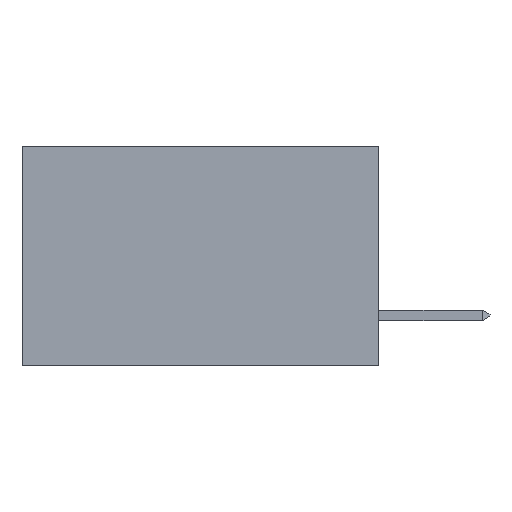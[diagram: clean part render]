
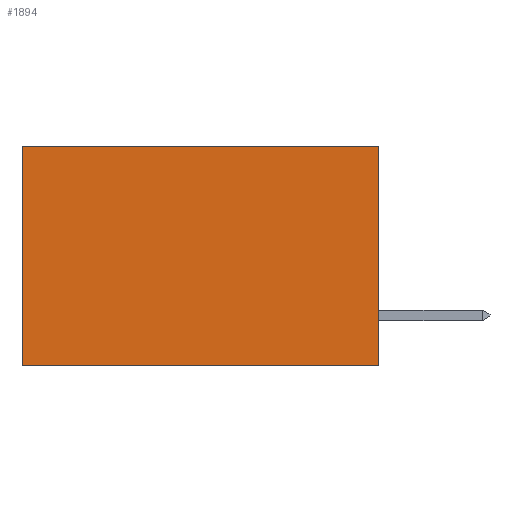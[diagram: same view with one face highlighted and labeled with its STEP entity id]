
A CAD part, left-side view. The second image highlights one B-rep face of the part: STEP entity #1894.
In plain terms, the highlighted planar face has unit normal (-1, 0, 0).
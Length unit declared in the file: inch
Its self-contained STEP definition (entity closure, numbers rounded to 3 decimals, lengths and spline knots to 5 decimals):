
#121 = DIRECTION ( 'NONE',  ( 0., 0., -1. ) ) ;
#759 = LINE ( 'NONE', #5815, #2661 ) ;
#812 = EDGE_CURVE ( 'NONE', #4451, #4891, #1941, .T. ) ;
#995 = ORIENTED_EDGE ( 'NONE', *, *, #5624, .F. ) ;
#1079 = DIRECTION ( 'NONE',  ( 0., 0., -1. ) ) ;
#1494 = VERTEX_POINT ( 'NONE', #2460 ) ;
#1613 = VECTOR ( 'NONE', #5376, 39.37008 ) ;
#1894 = ADVANCED_FACE ( 'NONE', ( #5546 ), #3663, .F. ) ;
#1941 = LINE ( 'NONE', #3827, #5171 ) ;
#2460 = CARTESIAN_POINT ( 'NONE',  ( 0.2615, 0.6, -0.37 ) ) ;
#2661 = VECTOR ( 'NONE', #121, 39.37008 ) ;
#2684 = CARTESIAN_POINT ( 'NONE',  ( 0.2615, 0.6, 0. ) ) ;
#2993 = CARTESIAN_POINT ( 'NONE',  ( 0.2615, 0., -0.37 ) ) ;
#3031 = ORIENTED_EDGE ( 'NONE', *, *, #812, .T. ) ;
#3555 = DIRECTION ( 'NONE',  ( 0., 0., -1. ) ) ;
#3663 = PLANE ( 'NONE',  #5714 ) ;
#3713 = CARTESIAN_POINT ( 'NONE',  ( 0.2615, 0., -0.37 ) ) ;
#3827 = CARTESIAN_POINT ( 'NONE',  ( 0.2615, 0., 0. ) ) ;
#3963 = EDGE_CURVE ( 'NONE', #4891, #1494, #759, .T. ) ;
#4147 = LINE ( 'NONE', #4719, #1613 ) ;
#4451 = VERTEX_POINT ( 'NONE', #6753 ) ;
#4480 = DIRECTION ( 'NONE',  ( 0., 1., 0. ) ) ;
#4518 = VECTOR ( 'NONE', #3555, 39.37008 ) ;
#4719 = CARTESIAN_POINT ( 'NONE',  ( 0.2615, 0., -0.37 ) ) ;
#4883 = DIRECTION ( 'NONE',  ( 1., 0., 0. ) ) ;
#4891 = VERTEX_POINT ( 'NONE', #2684 ) ;
#5100 = VERTEX_POINT ( 'NONE', #7742 ) ;
#5171 = VECTOR ( 'NONE', #4480, 39.37008 ) ;
#5376 = DIRECTION ( 'NONE',  ( 0., 1., 0. ) ) ;
#5419 = ORIENTED_EDGE ( 'NONE', *, *, #3963, .T. ) ;
#5546 = FACE_OUTER_BOUND ( 'NONE', #7747, .T. ) ;
#5624 = EDGE_CURVE ( 'NONE', #4451, #5100, #6069, .T. ) ;
#5714 = AXIS2_PLACEMENT_3D ( 'NONE', #2993, #4883, #1079 ) ;
#5815 = CARTESIAN_POINT ( 'NONE',  ( 0.2615, 0.6, -0.37 ) ) ;
#5992 = ORIENTED_EDGE ( 'NONE', *, *, #6384, .F. ) ;
#6069 = LINE ( 'NONE', #3713, #4518 ) ;
#6384 = EDGE_CURVE ( 'NONE', #5100, #1494, #4147, .T. ) ;
#6753 = CARTESIAN_POINT ( 'NONE',  ( 0.2615, 0., 0. ) ) ;
#7742 = CARTESIAN_POINT ( 'NONE',  ( 0.2615, 0., -0.37 ) ) ;
#7747 = EDGE_LOOP ( 'NONE', ( #5419, #5992, #995, #3031 ) ) ;
